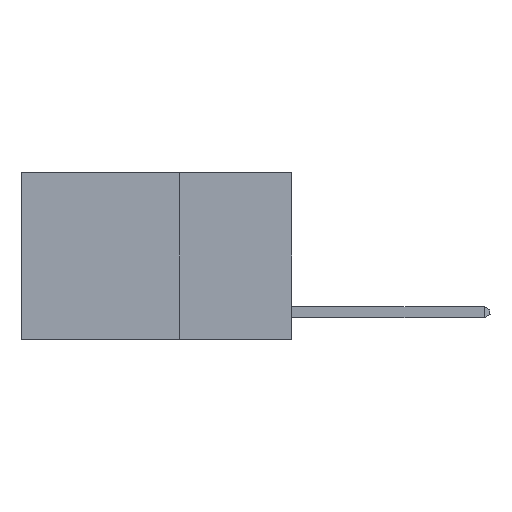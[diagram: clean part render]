
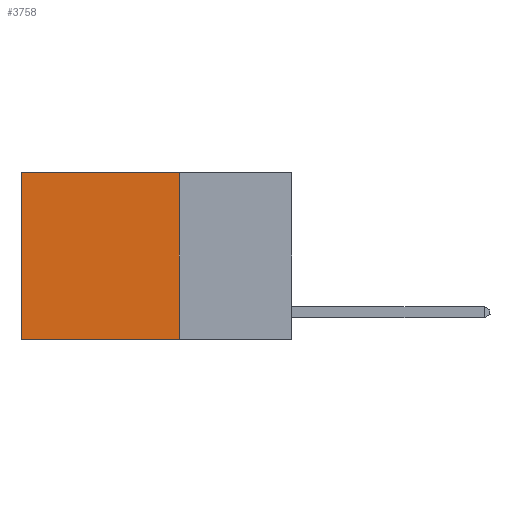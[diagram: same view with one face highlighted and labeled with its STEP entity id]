
A CAD part, left-side view. The second image highlights one B-rep face of the part: STEP entity #3758.
In plain terms, the highlighted planar face has unit normal (-1, 0, 0).
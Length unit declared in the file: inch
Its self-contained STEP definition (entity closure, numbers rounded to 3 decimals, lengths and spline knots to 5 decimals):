
#126 = EDGE_CURVE ( 'NONE', #7766, #2097, #4482, .T. ) ;
#337 = VECTOR ( 'NONE', #5431, 39.37008 ) ;
#671 = ORIENTED_EDGE ( 'NONE', *, *, #10986, .T. ) ;
#709 = CARTESIAN_POINT ( 'NONE',  ( 0.2625, 0.25, 0. ) ) ;
#1099 = DIRECTION ( 'NONE',  ( 0., 0., -1. ) ) ;
#1171 = AXIS2_PLACEMENT_3D ( 'NONE', #9321, #10463, #3748 ) ;
#2097 = VERTEX_POINT ( 'NONE', #10052 ) ;
#2106 = EDGE_CURVE ( 'NONE', #7766, #5161, #10411, .T. ) ;
#2107 = VERTEX_POINT ( 'NONE', #4457 ) ;
#2113 = DIRECTION ( 'NONE',  ( 0., 1., 0. ) ) ;
#2492 = ORIENTED_EDGE ( 'NONE', *, *, #126, .T. ) ;
#2660 = ORIENTED_EDGE ( 'NONE', *, *, #2106, .F. ) ;
#3034 = LINE ( 'NONE', #9879, #337 ) ;
#3748 = DIRECTION ( 'NONE',  ( 0., 0., -1. ) ) ;
#3758 = ADVANCED_FACE ( 'NONE', ( #7123 ), #13822, .F. ) ;
#3819 = EDGE_CURVE ( 'NONE', #5161, #2107, #12060, .T. ) ;
#4457 = CARTESIAN_POINT ( 'NONE',  ( 0.2625, 0.6, -0.37 ) ) ;
#4482 = LINE ( 'NONE', #709, #11148 ) ;
#5161 = VERTEX_POINT ( 'NONE', #6244 ) ;
#5431 = DIRECTION ( 'NONE',  ( 0., 0., -1. ) ) ;
#5582 = EDGE_LOOP ( 'NONE', ( #671, #14458, #2660, #2492 ) ) ;
#6244 = CARTESIAN_POINT ( 'NONE',  ( 0.2625, 0.25, -0.37 ) ) ;
#7123 = FACE_OUTER_BOUND ( 'NONE', #5582, .T. ) ;
#7766 = VERTEX_POINT ( 'NONE', #12969 ) ;
#9321 = CARTESIAN_POINT ( 'NONE',  ( 0.2625, 0.25, 0. ) ) ;
#9879 = CARTESIAN_POINT ( 'NONE',  ( 0.2625, 0.6, 0. ) ) ;
#10052 = CARTESIAN_POINT ( 'NONE',  ( 0.2625, 0.6, 0. ) ) ;
#10064 = VECTOR ( 'NONE', #1099, 39.37008 ) ;
#10411 = LINE ( 'NONE', #12320, #10064 ) ;
#10463 = DIRECTION ( 'NONE',  ( 1., 0., 0. ) ) ;
#10986 = EDGE_CURVE ( 'NONE', #2097, #2107, #3034, .T. ) ;
#11148 = VECTOR ( 'NONE', #2113, 39.37008 ) ;
#11699 = CARTESIAN_POINT ( 'NONE',  ( 0.2625, 0.25, -0.37 ) ) ;
#11708 = VECTOR ( 'NONE', #13919, 39.37008 ) ;
#12060 = LINE ( 'NONE', #11699, #11708 ) ;
#12320 = CARTESIAN_POINT ( 'NONE',  ( 0.2625, 0.25, 0. ) ) ;
#12969 = CARTESIAN_POINT ( 'NONE',  ( 0.2625, 0.25, 0. ) ) ;
#13822 = PLANE ( 'NONE',  #1171 ) ;
#13919 = DIRECTION ( 'NONE',  ( 0., 1., 0. ) ) ;
#14458 = ORIENTED_EDGE ( 'NONE', *, *, #3819, .F. ) ;
